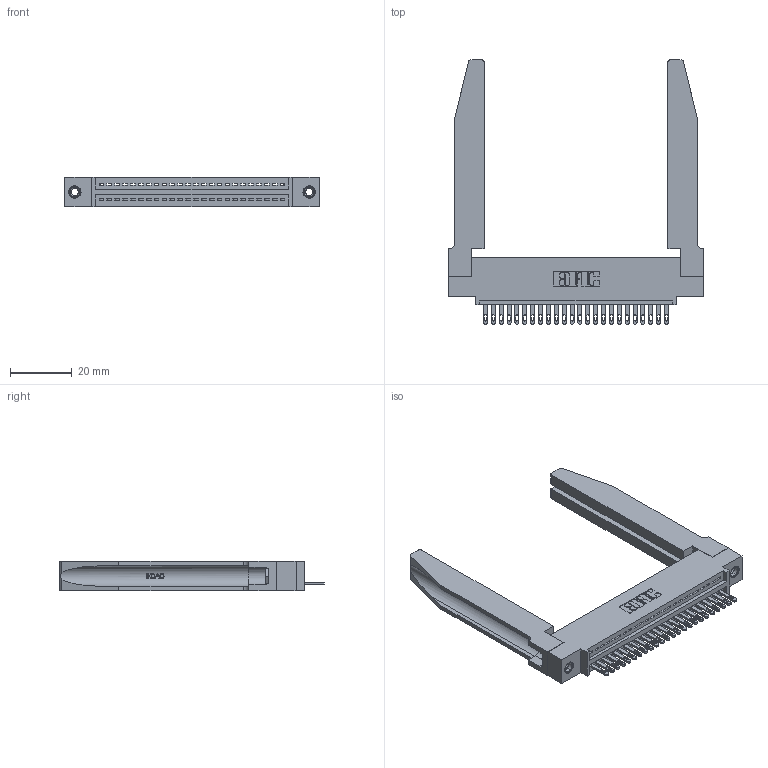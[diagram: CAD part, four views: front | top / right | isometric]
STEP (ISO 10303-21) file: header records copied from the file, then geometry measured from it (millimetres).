
FILE_DESCRIPTION (( 'STEP AP203' ), '1' );
FILE_NAME ('345-024-500-478.STEP', '2019-10-05T03:32:11', ( '' ), ( '' ), 'SwSTEP 2.0', 'SolidWorks 2016', '' );
FILE_SCHEMA (( 'CONFIG_CONTROL_DESIGN' ));
Length unit declared in the file: inch
Products named in the file (5): 345-250-001_345-250-001-102; 345-220-078_345-220-078; 345 Part_0.110 Offset - 0.156 Dia-TH; 345-024-500-478; 345-292-001_345-293-100
Assembly tree (29 placements, depth 2):
  345-024-500-478
    345 Part_0.110 Offset - 0.156 Dia-TH
    345-292-001_345-293-100  x24
    345-250-001_345-250-001-102  x2
    345-220-078_345-220-078  x2
Bounding box: 82.19 x 85.27 x 9.4 mm (x, y, z)
Volume: 15371.4 mm3; surface area: 16837.7 mm2
Topology: 29 solids, 29 shells, 1660 faces, 4993 edges, 3318 vertices
Faces by surface type: plane 1042, cylinder 566, bspline 36, cone 12, torus 4
Entity records: 25288 total; most frequent: CARTESIAN_POINT 5279, ORIENTED_EDGE 4134, DIRECTION 3645, EDGE_CURVE 2067, LINE 1741, VECTOR 1741, VERTEX_POINT 1372, AXIS2_PLACEMENT_3D 952
